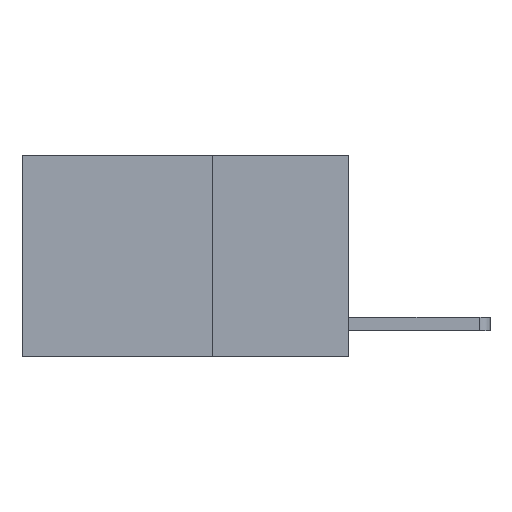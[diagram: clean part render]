
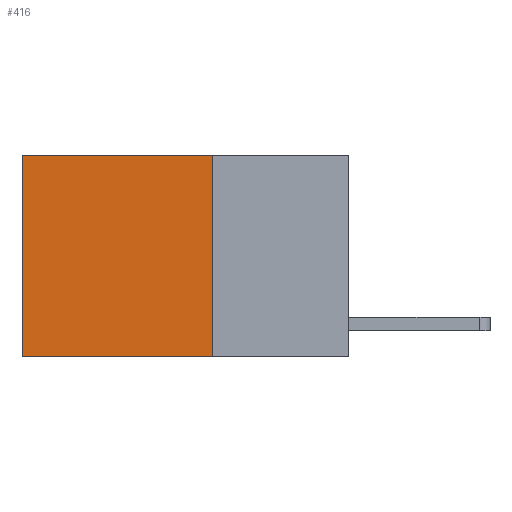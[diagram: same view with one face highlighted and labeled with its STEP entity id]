
A CAD part, left-side view. The second image highlights one B-rep face of the part: STEP entity #416.
In plain terms, the highlighted planar face has unit normal (-1, 0, 0).
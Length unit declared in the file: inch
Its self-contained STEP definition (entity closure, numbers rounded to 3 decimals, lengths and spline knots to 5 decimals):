
#134 = DIRECTION ( 'NONE',  ( 1., 0., 0. ) ) ;
#416 = ADVANCED_FACE ( 'NONE', ( #7247 ), #594, .F. ) ;
#552 = CARTESIAN_POINT ( 'NONE',  ( 0.2625, 0.25, -0.37 ) ) ;
#594 = PLANE ( 'NONE',  #8923 ) ;
#683 = ORIENTED_EDGE ( 'NONE', *, *, #5565, .F. ) ;
#879 = VECTOR ( 'NONE', #5030, 39.37008 ) ;
#950 = VECTOR ( 'NONE', #3669, 39.37008 ) ;
#974 = LINE ( 'NONE', #5054, #879 ) ;
#1058 = LINE ( 'NONE', #552, #950 ) ;
#1084 = ORIENTED_EDGE ( 'NONE', *, *, #4507, .T. ) ;
#1519 = DIRECTION ( 'NONE',  ( 0., 1., 0. ) ) ;
#1579 = CARTESIAN_POINT ( 'NONE',  ( 0.2625, 0.25, 0. ) ) ;
#1615 = ORIENTED_EDGE ( 'NONE', *, *, #4999, .F. ) ;
#2619 = VERTEX_POINT ( 'NONE', #7605 ) ;
#3206 = VERTEX_POINT ( 'NONE', #8847 ) ;
#3362 = CARTESIAN_POINT ( 'NONE',  ( 0.2625, 0.25, 0. ) ) ;
#3384 = DIRECTION ( 'NONE',  ( 0., 0., -1. ) ) ;
#3669 = DIRECTION ( 'NONE',  ( 0., 1., 0. ) ) ;
#3870 = EDGE_CURVE ( 'NONE', #7459, #3206, #974, .T. ) ;
#4041 = CARTESIAN_POINT ( 'NONE',  ( 0.2625, 0.25, 0. ) ) ;
#4507 = EDGE_CURVE ( 'NONE', #5475, #7459, #5787, .T. ) ;
#4598 = VECTOR ( 'NONE', #6231, 39.37008 ) ;
#4999 = EDGE_CURVE ( 'NONE', #2619, #3206, #1058, .T. ) ;
#5030 = DIRECTION ( 'NONE',  ( 0., 0., -1. ) ) ;
#5054 = CARTESIAN_POINT ( 'NONE',  ( 0.2625, 0.6, 0. ) ) ;
#5286 = CARTESIAN_POINT ( 'NONE',  ( 0.2625, 0.25, 0. ) ) ;
#5424 = VECTOR ( 'NONE', #1519, 39.37008 ) ;
#5475 = VERTEX_POINT ( 'NONE', #4041 ) ;
#5565 = EDGE_CURVE ( 'NONE', #5475, #2619, #6747, .T. ) ;
#5787 = LINE ( 'NONE', #1579, #5424 ) ;
#6231 = DIRECTION ( 'NONE',  ( 0., 0., -1. ) ) ;
#6747 = LINE ( 'NONE', #3362, #4598 ) ;
#7247 = FACE_OUTER_BOUND ( 'NONE', #7928, .T. ) ;
#7459 = VERTEX_POINT ( 'NONE', #8629 ) ;
#7605 = CARTESIAN_POINT ( 'NONE',  ( 0.2625, 0.25, -0.37 ) ) ;
#7928 = EDGE_LOOP ( 'NONE', ( #8697, #1615, #683, #1084 ) ) ;
#8629 = CARTESIAN_POINT ( 'NONE',  ( 0.2625, 0.6, 0. ) ) ;
#8697 = ORIENTED_EDGE ( 'NONE', *, *, #3870, .T. ) ;
#8847 = CARTESIAN_POINT ( 'NONE',  ( 0.2625, 0.6, -0.37 ) ) ;
#8923 = AXIS2_PLACEMENT_3D ( 'NONE', #5286, #134, #3384 ) ;
